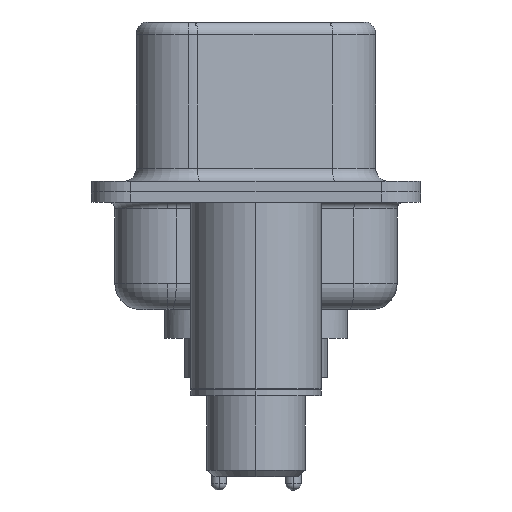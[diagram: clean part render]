
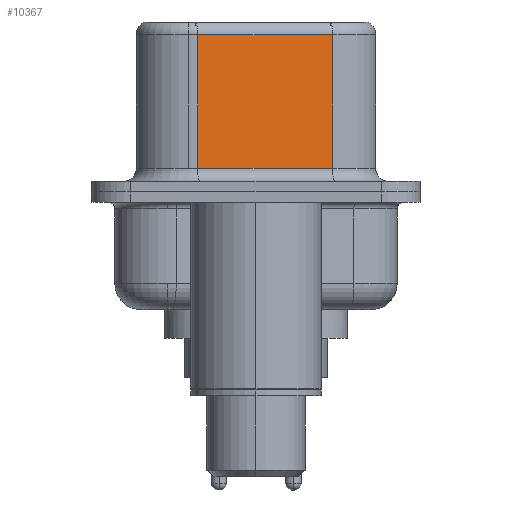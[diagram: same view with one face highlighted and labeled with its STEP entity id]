
A CAD part, left-side view. The second image highlights one B-rep face of the part: STEP entity #10367.
In plain terms, the highlighted planar face has unit normal (-0.985, -0.174, 0).
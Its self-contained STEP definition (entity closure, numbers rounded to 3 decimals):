
#1381 = CARTESIAN_POINT ( 'NONE',  ( 3.67, 2.233, 6.02 ) ) ;
#1413 = VERTEX_POINT ( 'NONE', #16669 ) ;
#2748 = CARTESIAN_POINT ( 'NONE',  ( 4.58, -2.927, 6.02 ) ) ;
#2992 = ORIENTED_EDGE ( 'NONE', *, *, #11529, .T. ) ;
#3490 = CARTESIAN_POINT ( 'NONE',  ( 4.58, -2.927, 6.52 ) ) ;
#4812 = DIRECTION ( 'NONE',  ( 0., 0., -1. ) ) ;
#6188 = VECTOR ( 'NONE', #16704, 1000. ) ;
#6321 = VECTOR ( 'NONE', #4812, 1000. ) ;
#6619 = EDGE_CURVE ( 'NONE', #1413, #18050, #17417, .T. ) ;
#6713 = FACE_OUTER_BOUND ( 'NONE', #21708, .T. ) ;
#8129 = VERTEX_POINT ( 'NONE', #24101 ) ;
#9214 = ORIENTED_EDGE ( 'NONE', *, *, #6619, .T. ) ;
#9660 = PLANE ( 'NONE',  #23882 ) ;
#9676 = LINE ( 'NONE', #24795, #23697 ) ;
#10367 = ADVANCED_FACE ( 'NONE', ( #6713 ), #9660, .F. ) ;
#11171 = DIRECTION ( 'NONE',  ( 0.174, -0.985, 0. ) ) ;
#11529 = EDGE_CURVE ( 'NONE', #8129, #17006, #9676, .T. ) ;
#13258 = DIRECTION ( 'NONE',  ( 0., 0., -1. ) ) ;
#13264 = LINE ( 'NONE', #3490, #17333 ) ;
#13292 = CARTESIAN_POINT ( 'NONE',  ( 4.58, -2.927, 6.52 ) ) ;
#14674 = CARTESIAN_POINT ( 'NONE',  ( 3.67, 2.233, 6.52 ) ) ;
#15532 = CARTESIAN_POINT ( 'NONE',  ( 4.58, -2.927, 0.9 ) ) ;
#15806 = DIRECTION ( 'NONE',  ( 0.985, 0.174, 0. ) ) ;
#16293 = LINE ( 'NONE', #14674, #6321 ) ;
#16669 = CARTESIAN_POINT ( 'NONE',  ( 4.58, -2.927, 6.02 ) ) ;
#16704 = DIRECTION ( 'NONE',  ( -0.174, 0.985, 0. ) ) ;
#17006 = VERTEX_POINT ( 'NONE', #15532 ) ;
#17333 = VECTOR ( 'NONE', #13258, 1000. ) ;
#17417 = LINE ( 'NONE', #2748, #6188 ) ;
#18050 = VERTEX_POINT ( 'NONE', #1381 ) ;
#18390 = EDGE_CURVE ( 'NONE', #18050, #8129, #16293, .T. ) ;
#21708 = EDGE_LOOP ( 'NONE', ( #21750, #9214, #23377, #2992 ) ) ;
#21750 = ORIENTED_EDGE ( 'NONE', *, *, #24774, .F. ) ;
#23377 = ORIENTED_EDGE ( 'NONE', *, *, #18390, .T. ) ;
#23697 = VECTOR ( 'NONE', #11171, 1000. ) ;
#23882 = AXIS2_PLACEMENT_3D ( 'NONE', #13292, #15806, #23923 ) ;
#23923 = DIRECTION ( 'NONE',  ( -0.174, 0.985, 0. ) ) ;
#24101 = CARTESIAN_POINT ( 'NONE',  ( 3.67, 2.233, 0.9 ) ) ;
#24774 = EDGE_CURVE ( 'NONE', #1413, #17006, #13264, .T. ) ;
#24795 = CARTESIAN_POINT ( 'NONE',  ( 4.58, -2.927, 0.9 ) ) ;
